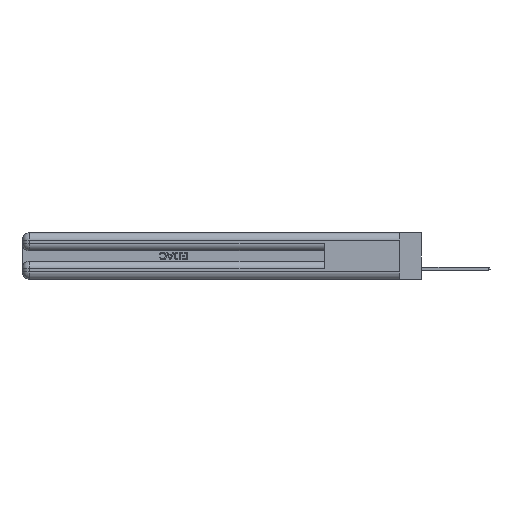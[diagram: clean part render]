
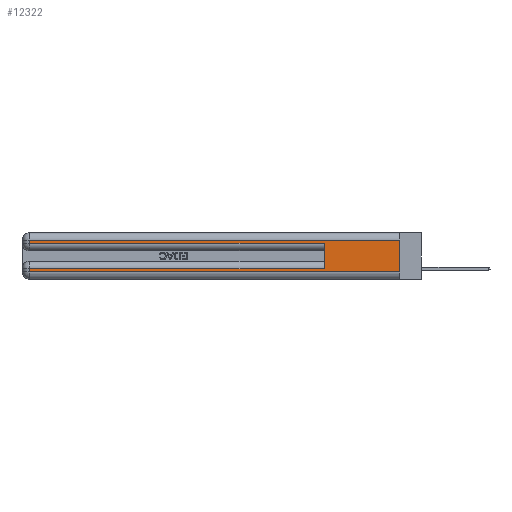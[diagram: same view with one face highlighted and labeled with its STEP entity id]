
A CAD part, left-side view. The second image highlights one B-rep face of the part: STEP entity #12322.
In plain terms, the highlighted planar face has unit normal (-1, 0, 0).
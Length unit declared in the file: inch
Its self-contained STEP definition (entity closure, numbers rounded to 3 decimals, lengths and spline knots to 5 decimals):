
#865 = VERTEX_POINT ( 'NONE', #38310 ) ;
#870 = EDGE_LOOP ( 'NONE', ( #31787, #42030, #51829, #20994, #31426, #11492, #50344, #15365 ) ) ;
#2594 = DIRECTION ( 'NONE',  ( 1., 0., 0. ) ) ;
#4114 = CARTESIAN_POINT ( 'NONE',  ( 0., 2.94, 0.37 ) ) ;
#8263 = EDGE_CURVE ( 'NONE', #48287, #865, #43428, .T. ) ;
#8352 = LINE ( 'NONE', #38790, #20666 ) ;
#9735 = CARTESIAN_POINT ( 'NONE',  ( 0., 0.6, 0.085 ) ) ;
#9992 = VECTOR ( 'NONE', #35437, 39.37008 ) ;
#11492 = ORIENTED_EDGE ( 'NONE', *, *, #43765, .T. ) ;
#12322 = ADVANCED_FACE ( 'NONE', ( #24424 ), #27383, .F. ) ;
#13030 = EDGE_CURVE ( 'NONE', #865, #36420, #26929, .T. ) ;
#14736 = CARTESIAN_POINT ( 'NONE',  ( 0., 0.6, 0.285 ) ) ;
#15238 = DIRECTION ( 'NONE',  ( 0., 0., -1. ) ) ;
#15365 = ORIENTED_EDGE ( 'NONE', *, *, #17622, .T. ) ;
#15585 = CARTESIAN_POINT ( 'NONE',  ( 0., 2.94, 0.06 ) ) ;
#15809 = CARTESIAN_POINT ( 'NONE',  ( 0., 2.94, 0.37 ) ) ;
#17622 = EDGE_CURVE ( 'NONE', #47430, #20055, #32630, .T. ) ;
#17833 = LINE ( 'NONE', #15809, #30136 ) ;
#18026 = LINE ( 'NONE', #32855, #30350 ) ;
#18422 = LINE ( 'NONE', #23119, #9992 ) ;
#19814 = DIRECTION ( 'NONE',  ( 0., -1., 0. ) ) ;
#20055 = VERTEX_POINT ( 'NONE', #43883 ) ;
#20666 = VECTOR ( 'NONE', #53046, 39.37008 ) ;
#20994 = ORIENTED_EDGE ( 'NONE', *, *, #13030, .T. ) ;
#22006 = VERTEX_POINT ( 'NONE', #9735 ) ;
#23119 = CARTESIAN_POINT ( 'NONE',  ( 0., 0.6, 0.145 ) ) ;
#23384 = CARTESIAN_POINT ( 'NONE',  ( 0., 0., 0.37 ) ) ;
#24424 = FACE_OUTER_BOUND ( 'NONE', #870, .T. ) ;
#24435 = VERTEX_POINT ( 'NONE', #26890 ) ;
#26033 = VECTOR ( 'NONE', #43792, 39.37008 ) ;
#26890 = CARTESIAN_POINT ( 'NONE',  ( 0., 2.94, 0.085 ) ) ;
#26903 = EDGE_CURVE ( 'NONE', #52437, #20055, #8352, .T. ) ;
#26929 = LINE ( 'NONE', #32129, #50930 ) ;
#27383 = PLANE ( 'NONE',  #43750 ) ;
#29497 = CARTESIAN_POINT ( 'NONE',  ( 0., 0., 0.31 ) ) ;
#30136 = VECTOR ( 'NONE', #49667, 39.37008 ) ;
#30350 = VECTOR ( 'NONE', #45915, 39.37008 ) ;
#31426 = ORIENTED_EDGE ( 'NONE', *, *, #39141, .F. ) ;
#31787 = ORIENTED_EDGE ( 'NONE', *, *, #26903, .F. ) ;
#32129 = CARTESIAN_POINT ( 'NONE',  ( 0., 0., 0.285 ) ) ;
#32630 = LINE ( 'NONE', #41412, #52064 ) ;
#32855 = CARTESIAN_POINT ( 'NONE',  ( 0., 0., 0.085 ) ) ;
#33915 = EDGE_CURVE ( 'NONE', #52437, #48287, #38393, .T. ) ;
#35437 = DIRECTION ( 'NONE',  ( 0., 0., 1. ) ) ;
#36420 = VERTEX_POINT ( 'NONE', #14736 ) ;
#36911 = VECTOR ( 'NONE', #45046, 39.37008 ) ;
#38310 = CARTESIAN_POINT ( 'NONE',  ( 0., 2.94, 0.285 ) ) ;
#38393 = LINE ( 'NONE', #43097, #26033 ) ;
#38790 = CARTESIAN_POINT ( 'NONE',  ( 0., 0., 0.37 ) ) ;
#39141 = EDGE_CURVE ( 'NONE', #22006, #36420, #18422, .T. ) ;
#41412 = CARTESIAN_POINT ( 'NONE',  ( 0., 0., 0.06 ) ) ;
#42030 = ORIENTED_EDGE ( 'NONE', *, *, #33915, .T. ) ;
#42525 = CARTESIAN_POINT ( 'NONE',  ( 0., 2.94, 0.31 ) ) ;
#43097 = CARTESIAN_POINT ( 'NONE',  ( 0., 0., 0.31 ) ) ;
#43428 = LINE ( 'NONE', #4114, #36911 ) ;
#43750 = AXIS2_PLACEMENT_3D ( 'NONE', #23384, #2594, #15238 ) ;
#43765 = EDGE_CURVE ( 'NONE', #22006, #24435, #18026, .T. ) ;
#43792 = DIRECTION ( 'NONE',  ( 0., 1., 0. ) ) ;
#43883 = CARTESIAN_POINT ( 'NONE',  ( 0., 0., 0.06 ) ) ;
#45046 = DIRECTION ( 'NONE',  ( 0., 0., -1. ) ) ;
#45170 = EDGE_CURVE ( 'NONE', #24435, #47430, #17833, .T. ) ;
#45217 = DIRECTION ( 'NONE',  ( 0., -1., 0. ) ) ;
#45915 = DIRECTION ( 'NONE',  ( 0., 1., 0. ) ) ;
#47430 = VERTEX_POINT ( 'NONE', #15585 ) ;
#48287 = VERTEX_POINT ( 'NONE', #42525 ) ;
#49667 = DIRECTION ( 'NONE',  ( 0., 0., -1. ) ) ;
#50344 = ORIENTED_EDGE ( 'NONE', *, *, #45170, .T. ) ;
#50930 = VECTOR ( 'NONE', #19814, 39.37008 ) ;
#51829 = ORIENTED_EDGE ( 'NONE', *, *, #8263, .T. ) ;
#52064 = VECTOR ( 'NONE', #45217, 39.37008 ) ;
#52437 = VERTEX_POINT ( 'NONE', #29497 ) ;
#53046 = DIRECTION ( 'NONE',  ( 0., 0., -1. ) ) ;
